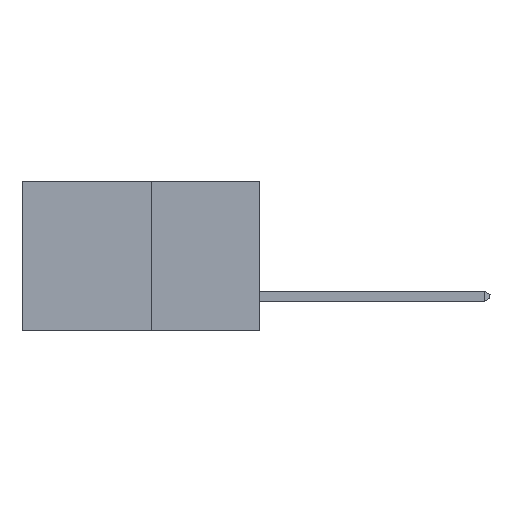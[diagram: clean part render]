
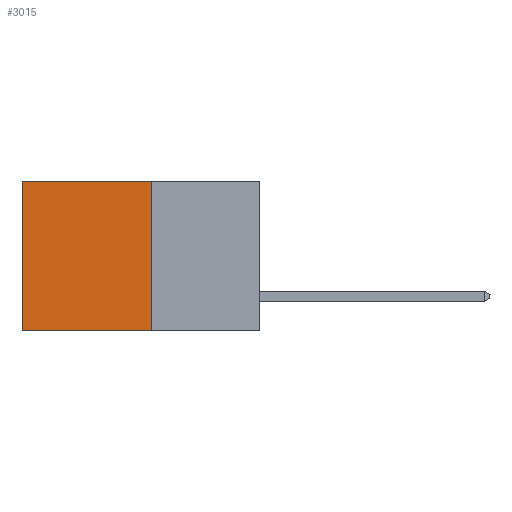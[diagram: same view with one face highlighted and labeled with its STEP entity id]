
A CAD part, left-side view. The second image highlights one B-rep face of the part: STEP entity #3015.
In plain terms, the highlighted planar face has unit normal (-1, 0, 0).
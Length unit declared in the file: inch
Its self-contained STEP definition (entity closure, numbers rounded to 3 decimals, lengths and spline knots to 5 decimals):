
#708 = LINE ( 'NONE', #7311, #5065 ) ;
#1529 = VERTEX_POINT ( 'NONE', #3214 ) ;
#1711 = VERTEX_POINT ( 'NONE', #10167 ) ;
#1793 = DIRECTION ( 'NONE',  ( 0., 1., 0. ) ) ;
#2213 = CARTESIAN_POINT ( 'NONE',  ( 0.277, 0.27, -0.37 ) ) ;
#2550 = EDGE_LOOP ( 'NONE', ( #10725, #10778, #10488, #10212 ) ) ;
#2806 = EDGE_CURVE ( 'NONE', #9514, #1529, #6592, .T. ) ;
#2879 = CARTESIAN_POINT ( 'NONE',  ( 0.277, 0.27, -0.37 ) ) ;
#2893 = DIRECTION ( 'NONE',  ( 0., 0., -1. ) ) ;
#3015 = ADVANCED_FACE ( 'NONE', ( #7657 ), #7804, .F. ) ;
#3214 = CARTESIAN_POINT ( 'NONE',  ( 0.277, 0.59, -0.37 ) ) ;
#3287 = LINE ( 'NONE', #2879, #9687 ) ;
#4293 = DIRECTION ( 'NONE',  ( 0., 1., 0. ) ) ;
#4362 = CARTESIAN_POINT ( 'NONE',  ( 0.277, 0.59, 0. ) ) ;
#5065 = VECTOR ( 'NONE', #7363, 39.37008 ) ;
#6019 = CARTESIAN_POINT ( 'NONE',  ( 0.277, 0.27, 0. ) ) ;
#6570 = EDGE_CURVE ( 'NONE', #1711, #9514, #3287, .T. ) ;
#6592 = LINE ( 'NONE', #2213, #6833 ) ;
#6629 = EDGE_CURVE ( 'NONE', #7900, #1529, #708, .T. ) ;
#6833 = VECTOR ( 'NONE', #1793, 39.37008 ) ;
#7045 = EDGE_CURVE ( 'NONE', #1711, #7900, #7795, .T. ) ;
#7311 = CARTESIAN_POINT ( 'NONE',  ( 0.277, 0.59, -0.37 ) ) ;
#7363 = DIRECTION ( 'NONE',  ( 0., 0., -1. ) ) ;
#7537 = DIRECTION ( 'NONE',  ( 0., 0., -1. ) ) ;
#7550 = VECTOR ( 'NONE', #4293, 39.37008 ) ;
#7573 = DIRECTION ( 'NONE',  ( 1., 0., 0. ) ) ;
#7657 = FACE_OUTER_BOUND ( 'NONE', #2550, .T. ) ;
#7795 = LINE ( 'NONE', #6019, #7550 ) ;
#7804 = PLANE ( 'NONE',  #10923 ) ;
#7900 = VERTEX_POINT ( 'NONE', #4362 ) ;
#8027 = CARTESIAN_POINT ( 'NONE',  ( 0.277, 0.27, -0.37 ) ) ;
#9432 = CARTESIAN_POINT ( 'NONE',  ( 0.277, 0.27, -0.37 ) ) ;
#9514 = VERTEX_POINT ( 'NONE', #9432 ) ;
#9687 = VECTOR ( 'NONE', #2893, 39.37008 ) ;
#10167 = CARTESIAN_POINT ( 'NONE',  ( 0.277, 0.27, 0. ) ) ;
#10212 = ORIENTED_EDGE ( 'NONE', *, *, #7045, .T. ) ;
#10488 = ORIENTED_EDGE ( 'NONE', *, *, #6570, .F. ) ;
#10725 = ORIENTED_EDGE ( 'NONE', *, *, #6629, .T. ) ;
#10778 = ORIENTED_EDGE ( 'NONE', *, *, #2806, .F. ) ;
#10923 = AXIS2_PLACEMENT_3D ( 'NONE', #8027, #7573, #7537 ) ;
